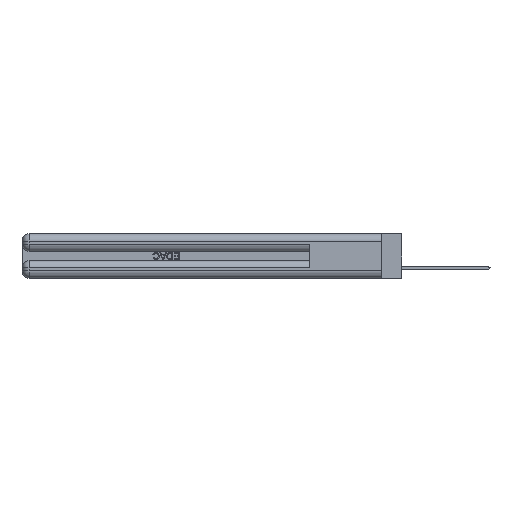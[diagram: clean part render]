
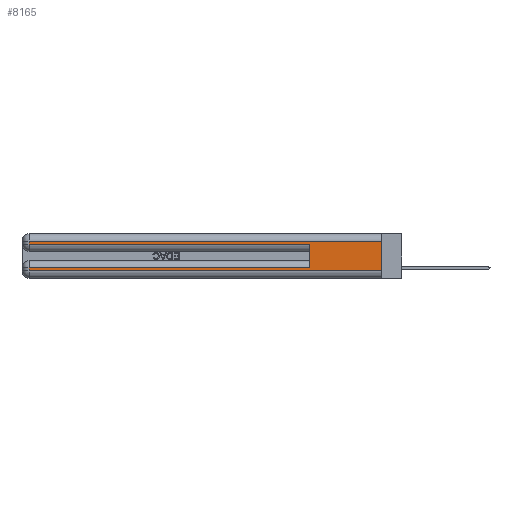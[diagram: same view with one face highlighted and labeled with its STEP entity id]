
A CAD part, left-side view. The second image highlights one B-rep face of the part: STEP entity #8165.
In plain terms, the highlighted planar face has unit normal (-1, 0, 0).
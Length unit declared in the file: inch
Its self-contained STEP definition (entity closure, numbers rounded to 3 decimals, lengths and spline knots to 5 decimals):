
#10 = ORIENTED_EDGE ( 'NONE', *, *, #6925, .T. ) ;
#544 = CARTESIAN_POINT ( 'NONE',  ( 0., 2.94, 0.37 ) ) ;
#890 = LINE ( 'NONE', #10889, #4259 ) ;
#1439 = LINE ( 'NONE', #16879, #51023 ) ;
#1912 = CARTESIAN_POINT ( 'NONE',  ( 0., 2.94, 0.31 ) ) ;
#4259 = VECTOR ( 'NONE', #23265, 39.37008 ) ;
#4762 = VECTOR ( 'NONE', #14681, 39.37008 ) ;
#5285 = CARTESIAN_POINT ( 'NONE',  ( 0., 0., 0.31 ) ) ;
#5523 = DIRECTION ( 'NONE',  ( 1., 0., 0. ) ) ;
#6373 = CARTESIAN_POINT ( 'NONE',  ( 0., 0., 0.31 ) ) ;
#6739 = VECTOR ( 'NONE', #38286, 39.37008 ) ;
#6925 = EDGE_CURVE ( 'NONE', #9612, #52240, #1439, .T. ) ;
#8165 = ADVANCED_FACE ( 'NONE', ( #49637 ), #26060, .F. ) ;
#8375 = ORIENTED_EDGE ( 'NONE', *, *, #14318, .T. ) ;
#9612 = VERTEX_POINT ( 'NONE', #41979 ) ;
#10889 = CARTESIAN_POINT ( 'NONE',  ( 0., 0., 0.37 ) ) ;
#11760 = ORIENTED_EDGE ( 'NONE', *, *, #28768, .T. ) ;
#12873 = EDGE_CURVE ( 'NONE', #52240, #15968, #31516, .T. ) ;
#13715 = CARTESIAN_POINT ( 'NONE',  ( 0., 0., 0.37 ) ) ;
#14079 = VECTOR ( 'NONE', #39746, 39.37008 ) ;
#14318 = EDGE_CURVE ( 'NONE', #22794, #15293, #31391, .T. ) ;
#14681 = DIRECTION ( 'NONE',  ( 0., 0., 1. ) ) ;
#15293 = VERTEX_POINT ( 'NONE', #1912 ) ;
#15968 = VERTEX_POINT ( 'NONE', #30818 ) ;
#16879 = CARTESIAN_POINT ( 'NONE',  ( 0., 2.94, 0.37 ) ) ;
#18379 = DIRECTION ( 'NONE',  ( 0., 1., 0. ) ) ;
#19020 = VERTEX_POINT ( 'NONE', #46106 ) ;
#20024 = VERTEX_POINT ( 'NONE', #36789 ) ;
#20341 = VECTOR ( 'NONE', #18379, 39.37008 ) ;
#22290 = LINE ( 'NONE', #544, #6739 ) ;
#22794 = VERTEX_POINT ( 'NONE', #6373 ) ;
#23115 = ORIENTED_EDGE ( 'NONE', *, *, #34101, .T. ) ;
#23265 = DIRECTION ( 'NONE',  ( 0., 0., -1. ) ) ;
#24463 = EDGE_CURVE ( 'NONE', #20024, #41299, #46472, .T. ) ;
#24941 = LINE ( 'NONE', #34803, #32811 ) ;
#25141 = LINE ( 'NONE', #32091, #14079 ) ;
#26060 = PLANE ( 'NONE',  #35741 ) ;
#28646 = CARTESIAN_POINT ( 'NONE',  ( 0., 0.6, 0.285 ) ) ;
#28768 = EDGE_CURVE ( 'NONE', #20024, #9612, #24941, .T. ) ;
#30818 = CARTESIAN_POINT ( 'NONE',  ( 0., 0., 0.06 ) ) ;
#30964 = DIRECTION ( 'NONE',  ( 0., 1., 0. ) ) ;
#31391 = LINE ( 'NONE', #5285, #20341 ) ;
#31516 = LINE ( 'NONE', #42088, #47844 ) ;
#32017 = ORIENTED_EDGE ( 'NONE', *, *, #12873, .T. ) ;
#32091 = CARTESIAN_POINT ( 'NONE',  ( 0., 0., 0.285 ) ) ;
#32811 = VECTOR ( 'NONE', #30964, 39.37008 ) ;
#34101 = EDGE_CURVE ( 'NONE', #19020, #41299, #25141, .T. ) ;
#34803 = CARTESIAN_POINT ( 'NONE',  ( 0., 0., 0.085 ) ) ;
#35708 = EDGE_CURVE ( 'NONE', #15293, #19020, #22290, .T. ) ;
#35741 = AXIS2_PLACEMENT_3D ( 'NONE', #13715, #5523, #36137 ) ;
#36137 = DIRECTION ( 'NONE',  ( 0., 0., -1. ) ) ;
#36789 = CARTESIAN_POINT ( 'NONE',  ( 0., 0.6, 0.085 ) ) ;
#37422 = ORIENTED_EDGE ( 'NONE', *, *, #24463, .F. ) ;
#37775 = ORIENTED_EDGE ( 'NONE', *, *, #43788, .F. ) ;
#38286 = DIRECTION ( 'NONE',  ( 0., 0., -1. ) ) ;
#39320 = CARTESIAN_POINT ( 'NONE',  ( 0., 2.94, 0.06 ) ) ;
#39509 = ORIENTED_EDGE ( 'NONE', *, *, #35708, .T. ) ;
#39746 = DIRECTION ( 'NONE',  ( 0., -1., 0. ) ) ;
#41299 = VERTEX_POINT ( 'NONE', #28646 ) ;
#41979 = CARTESIAN_POINT ( 'NONE',  ( 0., 2.94, 0.085 ) ) ;
#42088 = CARTESIAN_POINT ( 'NONE',  ( 0., 0., 0.06 ) ) ;
#43788 = EDGE_CURVE ( 'NONE', #22794, #15968, #890, .T. ) ;
#43858 = CARTESIAN_POINT ( 'NONE',  ( 0., 0.6, 0.145 ) ) ;
#46106 = CARTESIAN_POINT ( 'NONE',  ( 0., 2.94, 0.285 ) ) ;
#46472 = LINE ( 'NONE', #43858, #4762 ) ;
#47261 = DIRECTION ( 'NONE',  ( 0., 0., -1. ) ) ;
#47321 = EDGE_LOOP ( 'NONE', ( #37775, #8375, #39509, #23115, #37422, #11760, #10, #32017 ) ) ;
#47844 = VECTOR ( 'NONE', #50909, 39.37008 ) ;
#49637 = FACE_OUTER_BOUND ( 'NONE', #47321, .T. ) ;
#50909 = DIRECTION ( 'NONE',  ( 0., -1., 0. ) ) ;
#51023 = VECTOR ( 'NONE', #47261, 39.37008 ) ;
#52240 = VERTEX_POINT ( 'NONE', #39320 ) ;
